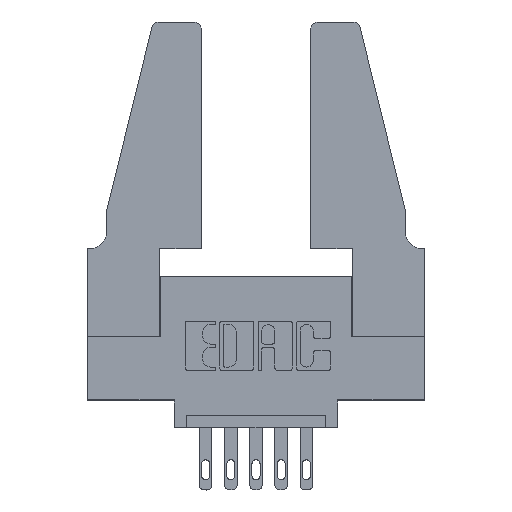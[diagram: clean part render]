
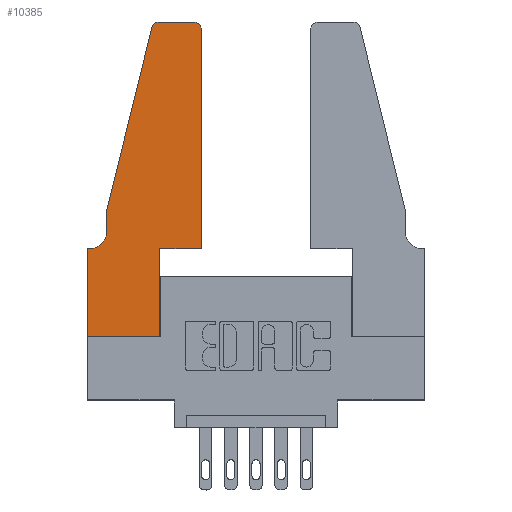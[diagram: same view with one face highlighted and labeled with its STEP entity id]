
A CAD part, top view. The second image highlights one B-rep face of the part: STEP entity #10385.
In plain terms, the highlighted planar face has unit normal (0, 0, 1).
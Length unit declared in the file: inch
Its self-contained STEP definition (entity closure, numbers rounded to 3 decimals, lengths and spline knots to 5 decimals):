
#79 = DIRECTION ( 'NONE',  ( 1., 0., 0. ) ) ;
#123 = CIRCLE ( 'NONE', #1636, 0.03 ) ;
#206 = VERTEX_POINT ( 'NONE', #662 ) ;
#227 = CARTESIAN_POINT ( 'NONE',  ( 0.4505, 0.35, 0.37 ) ) ;
#278 = AXIS2_PLACEMENT_3D ( 'NONE', #10896, #7617, #9319 ) ;
#384 = VERTEX_POINT ( 'NONE', #3432 ) ;
#438 = ORIENTED_EDGE ( 'NONE', *, *, #3612, .T. ) ;
#583 = DIRECTION ( 'NONE',  ( 0., -1., 0. ) ) ;
#623 = VERTEX_POINT ( 'NONE', #2046 ) ;
#635 = VECTOR ( 'NONE', #3321, 39.37008 ) ;
#662 = CARTESIAN_POINT ( 'NONE',  ( 0., 0., 0.37 ) ) ;
#738 = VERTEX_POINT ( 'NONE', #2284 ) ;
#743 = CARTESIAN_POINT ( 'NONE',  ( 0.4505, 1.22, 0.37 ) ) ;
#748 = ORIENTED_EDGE ( 'NONE', *, *, #2689, .T. ) ;
#934 = VECTOR ( 'NONE', #8265, 39.37008 ) ;
#1005 = CARTESIAN_POINT ( 'NONE',  ( 0.0755, 0.35, 0.37 ) ) ;
#1279 = ORIENTED_EDGE ( 'NONE', *, *, #1326, .T. ) ;
#1326 = EDGE_CURVE ( 'NONE', #9092, #7835, #3528, .T. ) ;
#1342 = EDGE_CURVE ( 'NONE', #8138, #3063, #5830, .T. ) ;
#1636 = AXIS2_PLACEMENT_3D ( 'NONE', #5738, #9080, #10912 ) ;
#1641 = DIRECTION ( 'NONE',  ( 0., 1., 0. ) ) ;
#1653 = DIRECTION ( 'NONE',  ( 0., 0., -1. ) ) ;
#1712 = VECTOR ( 'NONE', #1641, 39.37008 ) ;
#1765 = CIRCLE ( 'NONE', #278, 0.03 ) ;
#2046 = CARTESIAN_POINT ( 'NONE',  ( 0.2865, 0., 0.37 ) ) ;
#2095 = VERTEX_POINT ( 'NONE', #8264 ) ;
#2267 = ORIENTED_EDGE ( 'NONE', *, *, #3487, .T. ) ;
#2284 = CARTESIAN_POINT ( 'NONE',  ( 0.4205, 1.25, 0.37 ) ) ;
#2689 = EDGE_CURVE ( 'NONE', #738, #2095, #6493, .T. ) ;
#2693 = ORIENTED_EDGE ( 'NONE', *, *, #10116, .T. ) ;
#2790 = CARTESIAN_POINT ( 'NONE',  ( 0., 0.35, 0.37 ) ) ;
#2792 = LINE ( 'NONE', #10461, #10328 ) ;
#2889 = EDGE_CURVE ( 'NONE', #10171, #3461, #2792, .T. ) ;
#2954 = LINE ( 'NONE', #3531, #9424 ) ;
#3063 = VERTEX_POINT ( 'NONE', #9736 ) ;
#3158 = LINE ( 'NONE', #227, #10706 ) ;
#3214 = CARTESIAN_POINT ( 'NONE',  ( 0.2605, 1.25, 0.37 ) ) ;
#3321 = DIRECTION ( 'NONE',  ( 0., -1., 0. ) ) ;
#3341 = ORIENTED_EDGE ( 'NONE', *, *, #1342, .T. ) ;
#3432 = CARTESIAN_POINT ( 'NONE',  ( 0.2865, 0.35, 0.37 ) ) ;
#3461 = VERTEX_POINT ( 'NONE', #743 ) ;
#3487 = EDGE_CURVE ( 'NONE', #623, #384, #7391, .T. ) ;
#3528 = LINE ( 'NONE', #9224, #10002 ) ;
#3531 = CARTESIAN_POINT ( 'NONE',  ( 0., 0., 0.37 ) ) ;
#3532 = LINE ( 'NONE', #8194, #6830 ) ;
#3612 = EDGE_CURVE ( 'NONE', #384, #10171, #3158, .T. ) ;
#3909 = CARTESIAN_POINT ( 'NONE',  ( 0., 0.35, 0.37 ) ) ;
#4033 = CARTESIAN_POINT ( 'NONE',  ( 0.25487, 1.22718, 0.37 ) ) ;
#4059 = AXIS2_PLACEMENT_3D ( 'NONE', #10160, #1653, #10095 ) ;
#4404 = DIRECTION ( 'NONE',  ( 1., 0., 0. ) ) ;
#4449 = ORIENTED_EDGE ( 'NONE', *, *, #6913, .T. ) ;
#4601 = EDGE_CURVE ( 'NONE', #7835, #8138, #3532, .T. ) ;
#4613 = CARTESIAN_POINT ( 'NONE',  ( 0.4505, 0.35, 0.37 ) ) ;
#4971 = DIRECTION ( 'NONE',  ( -0.239, -0.971, 0. ) ) ;
#5126 = LINE ( 'NONE', #1005, #9215 ) ;
#5447 = ORIENTED_EDGE ( 'NONE', *, *, #10107, .T. ) ;
#5738 = CARTESIAN_POINT ( 'NONE',  ( 0.284, 1.22, 0.37 ) ) ;
#5830 = CIRCLE ( 'NONE', #4059, 0.07 ) ;
#5891 = CARTESIAN_POINT ( 'NONE',  ( 0.0755, 0.42, 0.37 ) ) ;
#5968 = CARTESIAN_POINT ( 'NONE',  ( 0.2865, 0.35, 0.37 ) ) ;
#6008 = VERTEX_POINT ( 'NONE', #2790 ) ;
#6493 = LINE ( 'NONE', #3214, #934 ) ;
#6723 = EDGE_CURVE ( 'NONE', #3461, #738, #1765, .T. ) ;
#6830 = VECTOR ( 'NONE', #583, 39.37008 ) ;
#6913 = EDGE_CURVE ( 'NONE', #206, #623, #2954, .T. ) ;
#6955 = AXIS2_PLACEMENT_3D ( 'NONE', #3909, #7307, #9002 ) ;
#7005 = ORIENTED_EDGE ( 'NONE', *, *, #6723, .T. ) ;
#7307 = DIRECTION ( 'NONE',  ( 0., 0., 1. ) ) ;
#7391 = LINE ( 'NONE', #5968, #1712 ) ;
#7617 = DIRECTION ( 'NONE',  ( 0., 0., 1. ) ) ;
#7677 = DIRECTION ( 'NONE',  ( -1., 0., 0. ) ) ;
#7835 = VERTEX_POINT ( 'NONE', #10793 ) ;
#7885 = ORIENTED_EDGE ( 'NONE', *, *, #8530, .T. ) ;
#7894 = FACE_OUTER_BOUND ( 'NONE', #7929, .T. ) ;
#7929 = EDGE_LOOP ( 'NONE', ( #748, #7885, #1279, #8028, #3341, #2693, #5447, #4449, #2267, #438, #10946, #7005 ) ) ;
#8028 = ORIENTED_EDGE ( 'NONE', *, *, #4601, .T. ) ;
#8138 = VERTEX_POINT ( 'NONE', #5891 ) ;
#8194 = CARTESIAN_POINT ( 'NONE',  ( 0.0755, 0.5, 0.37 ) ) ;
#8264 = CARTESIAN_POINT ( 'NONE',  ( 0.284, 1.25, 0.37 ) ) ;
#8265 = DIRECTION ( 'NONE',  ( -1., 0., 0. ) ) ;
#8376 = CARTESIAN_POINT ( 'NONE',  ( 0., 0., 0.37 ) ) ;
#8530 = EDGE_CURVE ( 'NONE', #2095, #9092, #123, .T. ) ;
#8864 = DIRECTION ( 'NONE',  ( 0., 1., 0. ) ) ;
#9002 = DIRECTION ( 'NONE',  ( 1., 0., 0. ) ) ;
#9080 = DIRECTION ( 'NONE',  ( 0., 0., 1. ) ) ;
#9092 = VERTEX_POINT ( 'NONE', #4033 ) ;
#9215 = VECTOR ( 'NONE', #7677, 39.37008 ) ;
#9224 = CARTESIAN_POINT ( 'NONE',  ( 0.0755, 0.5, 0.37 ) ) ;
#9319 = DIRECTION ( 'NONE',  ( 1., 0., 0. ) ) ;
#9424 = VECTOR ( 'NONE', #4404, 39.37008 ) ;
#9736 = CARTESIAN_POINT ( 'NONE',  ( 0.0055, 0.35, 0.37 ) ) ;
#9787 = PLANE ( 'NONE',  #6955 ) ;
#10002 = VECTOR ( 'NONE', #4971, 39.37008 ) ;
#10095 = DIRECTION ( 'NONE',  ( -1., 0., 0. ) ) ;
#10107 = EDGE_CURVE ( 'NONE', #6008, #206, #10947, .T. ) ;
#10116 = EDGE_CURVE ( 'NONE', #3063, #6008, #5126, .T. ) ;
#10160 = CARTESIAN_POINT ( 'NONE',  ( 0.0055, 0.42, 0.37 ) ) ;
#10171 = VERTEX_POINT ( 'NONE', #4613 ) ;
#10328 = VECTOR ( 'NONE', #8864, 39.37008 ) ;
#10385 = ADVANCED_FACE ( 'NONE', ( #7894 ), #9787, .T. ) ;
#10461 = CARTESIAN_POINT ( 'NONE',  ( 0.4505, 0.35, 0.37 ) ) ;
#10706 = VECTOR ( 'NONE', #79, 39.37008 ) ;
#10793 = CARTESIAN_POINT ( 'NONE',  ( 0.0755, 0.5, 0.37 ) ) ;
#10896 = CARTESIAN_POINT ( 'NONE',  ( 0.4205, 1.22, 0.37 ) ) ;
#10912 = DIRECTION ( 'NONE',  ( 1., 0., 0. ) ) ;
#10946 = ORIENTED_EDGE ( 'NONE', *, *, #2889, .T. ) ;
#10947 = LINE ( 'NONE', #8376, #635 ) ;
